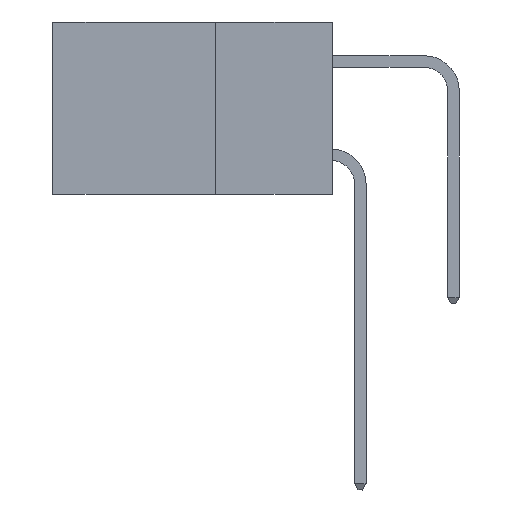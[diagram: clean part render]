
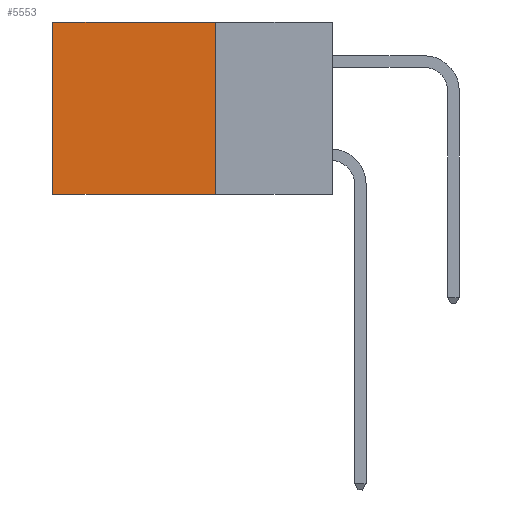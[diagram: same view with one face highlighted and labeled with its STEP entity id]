
A CAD part, left-side view. The second image highlights one B-rep face of the part: STEP entity #5553.
In plain terms, the highlighted planar face has unit normal (-1, 0, 0).
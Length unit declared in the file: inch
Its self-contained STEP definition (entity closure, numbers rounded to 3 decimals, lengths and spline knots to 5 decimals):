
#416 = PLANE ( 'NONE',  #4049 ) ;
#510 = ORIENTED_EDGE ( 'NONE', *, *, #11831, .T. ) ;
#629 = VECTOR ( 'NONE', #915, 39.37008 ) ;
#850 = LINE ( 'NONE', #10001, #3517 ) ;
#915 = DIRECTION ( 'NONE',  ( 0., 0., -1. ) ) ;
#1568 = DIRECTION ( 'NONE',  ( 0., 1., 0. ) ) ;
#1759 = CARTESIAN_POINT ( 'NONE',  ( 0.2615, 0.6, -0.37 ) ) ;
#1905 = EDGE_LOOP ( 'NONE', ( #510, #11848, #6271, #6716 ) ) ;
#2162 = CARTESIAN_POINT ( 'NONE',  ( 0.2615, 0.6, -0.37 ) ) ;
#2415 = CARTESIAN_POINT ( 'NONE',  ( 0.2615, 0.25, 0. ) ) ;
#2863 = VERTEX_POINT ( 'NONE', #2162 ) ;
#3027 = LINE ( 'NONE', #6570, #11471 ) ;
#3517 = VECTOR ( 'NONE', #4433, 39.37008 ) ;
#3822 = DIRECTION ( 'NONE',  ( 0., 0., -1. ) ) ;
#3940 = EDGE_CURVE ( 'NONE', #10482, #5268, #5304, .T. ) ;
#4049 = AXIS2_PLACEMENT_3D ( 'NONE', #4125, #10648, #9017 ) ;
#4125 = CARTESIAN_POINT ( 'NONE',  ( 0.2615, 0.25, -0.37 ) ) ;
#4433 = DIRECTION ( 'NONE',  ( 0., 1., 0. ) ) ;
#4808 = CARTESIAN_POINT ( 'NONE',  ( 0.2615, 0.6, 0. ) ) ;
#5268 = VERTEX_POINT ( 'NONE', #4808 ) ;
#5304 = LINE ( 'NONE', #9940, #6560 ) ;
#5495 = LINE ( 'NONE', #1759, #629 ) ;
#5515 = CARTESIAN_POINT ( 'NONE',  ( 0.2615, 0.25, -0.37 ) ) ;
#5553 = ADVANCED_FACE ( 'NONE', ( #8769 ), #416, .F. ) ;
#6271 = ORIENTED_EDGE ( 'NONE', *, *, #7697, .F. ) ;
#6560 = VECTOR ( 'NONE', #1568, 39.37008 ) ;
#6570 = CARTESIAN_POINT ( 'NONE',  ( 0.2615, 0.25, -0.37 ) ) ;
#6716 = ORIENTED_EDGE ( 'NONE', *, *, #3940, .T. ) ;
#7697 = EDGE_CURVE ( 'NONE', #10482, #11343, #3027, .T. ) ;
#8769 = FACE_OUTER_BOUND ( 'NONE', #1905, .T. ) ;
#8835 = EDGE_CURVE ( 'NONE', #11343, #2863, #850, .T. ) ;
#9017 = DIRECTION ( 'NONE',  ( 0., 0., -1. ) ) ;
#9940 = CARTESIAN_POINT ( 'NONE',  ( 0.2615, 0.25, 0. ) ) ;
#10001 = CARTESIAN_POINT ( 'NONE',  ( 0.2615, 0.25, -0.37 ) ) ;
#10482 = VERTEX_POINT ( 'NONE', #2415 ) ;
#10648 = DIRECTION ( 'NONE',  ( 1., 0., 0. ) ) ;
#11343 = VERTEX_POINT ( 'NONE', #5515 ) ;
#11471 = VECTOR ( 'NONE', #3822, 39.37008 ) ;
#11831 = EDGE_CURVE ( 'NONE', #5268, #2863, #5495, .T. ) ;
#11848 = ORIENTED_EDGE ( 'NONE', *, *, #8835, .F. ) ;
